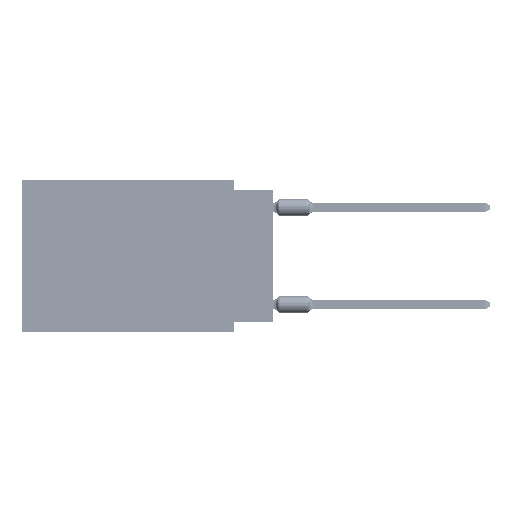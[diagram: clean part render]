
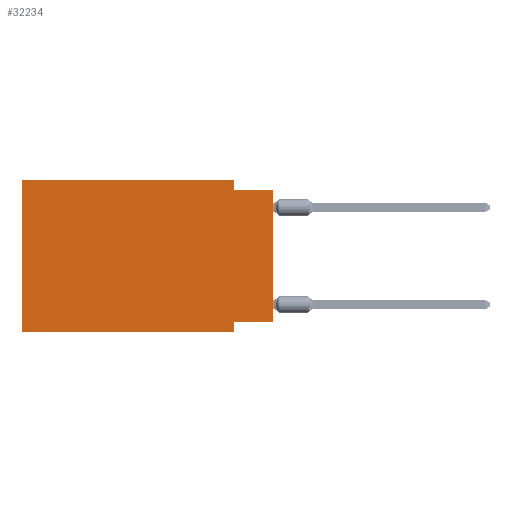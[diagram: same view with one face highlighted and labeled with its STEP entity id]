
A CAD part, left-side view. The second image highlights one B-rep face of the part: STEP entity #32234.
In plain terms, the highlighted planar face has unit normal (-1, 0, 0).
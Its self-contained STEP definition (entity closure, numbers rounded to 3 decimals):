
#1309 = CARTESIAN_POINT ( 'NONE',  ( 0., 2.54, -9.906 ) ) ;
#2368 = ORIENTED_EDGE ( 'NONE', *, *, #72979, .F. ) ;
#2607 = DIRECTION ( 'NONE',  ( 0., 0., -1. ) ) ;
#2869 = VERTEX_POINT ( 'NONE', #23513 ) ;
#4216 = EDGE_CURVE ( 'NONE', #22415, #53746, #67409, .T. ) ;
#5171 = DIRECTION ( 'NONE',  ( 0., 0., -1. ) ) ;
#5966 = CARTESIAN_POINT ( 'NONE',  ( 0., 16.383, -9.906 ) ) ;
#9535 = ORIENTED_EDGE ( 'NONE', *, *, #80196, .F. ) ;
#10734 = VERTEX_POINT ( 'NONE', #16359 ) ;
#12875 = EDGE_CURVE ( 'NONE', #22415, #37363, #29248, .T. ) ;
#15638 = CARTESIAN_POINT ( 'NONE',  ( 0., 2.54, 0. ) ) ;
#16359 = CARTESIAN_POINT ( 'NONE',  ( 0., 0., -0.635 ) ) ;
#18147 = EDGE_CURVE ( 'NONE', #49187, #87806, #49714, .T. ) ;
#18782 = VECTOR ( 'NONE', #42097, 1000. ) ;
#20379 = PLANE ( 'NONE',  #30728 ) ;
#22060 = VECTOR ( 'NONE', #2607, 1000. ) ;
#22415 = VERTEX_POINT ( 'NONE', #23471 ) ;
#23441 = CARTESIAN_POINT ( 'NONE',  ( 0., 2.54, -9.906 ) ) ;
#23471 = CARTESIAN_POINT ( 'NONE',  ( 0., 16.383, -9.906 ) ) ;
#23513 = CARTESIAN_POINT ( 'NONE',  ( 0., 0., -9.271 ) ) ;
#24281 = CARTESIAN_POINT ( 'NONE',  ( 0., 2.54, 0. ) ) ;
#25303 = DIRECTION ( 'NONE',  ( 0., -1., 0. ) ) ;
#26693 = FACE_OUTER_BOUND ( 'NONE', #75995, .T. ) ;
#29152 = ORIENTED_EDGE ( 'NONE', *, *, #18147, .F. ) ;
#29248 = LINE ( 'NONE', #64616, #82178 ) ;
#30728 = AXIS2_PLACEMENT_3D ( 'NONE', #54037, #39248, #5171 ) ;
#30742 = LINE ( 'NONE', #65251, #62306 ) ;
#32234 = ADVANCED_FACE ( 'NONE', ( #26693 ), #20379, .F. ) ;
#34248 = VECTOR ( 'NONE', #83323, 1000. ) ;
#35223 = ORIENTED_EDGE ( 'NONE', *, *, #56813, .T. ) ;
#35950 = DIRECTION ( 'NONE',  ( 0., 0., 1. ) ) ;
#37011 = DIRECTION ( 'NONE',  ( 0., -1., 0. ) ) ;
#37363 = VERTEX_POINT ( 'NONE', #61233 ) ;
#37779 = LINE ( 'NONE', #39539, #55965 ) ;
#39248 = DIRECTION ( 'NONE',  ( 1., 0., 0. ) ) ;
#39539 = CARTESIAN_POINT ( 'NONE',  ( 0., 0., 0. ) ) ;
#42097 = DIRECTION ( 'NONE',  ( 0., -1., 0. ) ) ;
#43469 = LINE ( 'NONE', #1309, #77709 ) ;
#45109 = CARTESIAN_POINT ( 'NONE',  ( 0., 2.54, -0.635 ) ) ;
#45384 = ORIENTED_EDGE ( 'NONE', *, *, #4216, .T. ) ;
#49187 = VERTEX_POINT ( 'NONE', #24281 ) ;
#49706 = CARTESIAN_POINT ( 'NONE',  ( 0., 0., -0.635 ) ) ;
#49714 = LINE ( 'NONE', #15638, #22060 ) ;
#52998 = DIRECTION ( 'NONE',  ( 0., 0., 1. ) ) ;
#53746 = VERTEX_POINT ( 'NONE', #23441 ) ;
#54037 = CARTESIAN_POINT ( 'NONE',  ( 0., 16.383, 0. ) ) ;
#55712 = EDGE_CURVE ( 'NONE', #87806, #10734, #77068, .T. ) ;
#55965 = VECTOR ( 'NONE', #52998, 1000. ) ;
#56813 = EDGE_CURVE ( 'NONE', #2869, #10734, #37779, .T. ) ;
#59453 = VECTOR ( 'NONE', #25303, 1000. ) ;
#61233 = CARTESIAN_POINT ( 'NONE',  ( 0., 16.383, 0. ) ) ;
#62306 = VECTOR ( 'NONE', #37011, 1000. ) ;
#62713 = LINE ( 'NONE', #84209, #34248 ) ;
#64616 = CARTESIAN_POINT ( 'NONE',  ( 0., 16.383, 0. ) ) ;
#65251 = CARTESIAN_POINT ( 'NONE',  ( 0., 16.383, 0. ) ) ;
#67409 = LINE ( 'NONE', #5966, #59453 ) ;
#67891 = ORIENTED_EDGE ( 'NONE', *, *, #12875, .F. ) ;
#72979 = EDGE_CURVE ( 'NONE', #2869, #83261, #62713, .T. ) ;
#74254 = ORIENTED_EDGE ( 'NONE', *, *, #76981, .F. ) ;
#74297 = ORIENTED_EDGE ( 'NONE', *, *, #55712, .F. ) ;
#75995 = EDGE_LOOP ( 'NONE', ( #35223, #74297, #29152, #9535, #67891, #45384, #74254, #2368 ) ) ;
#76754 = CARTESIAN_POINT ( 'NONE',  ( 0., 2.54, -9.271 ) ) ;
#76981 = EDGE_CURVE ( 'NONE', #83261, #53746, #43469, .T. ) ;
#77068 = LINE ( 'NONE', #49706, #18782 ) ;
#77709 = VECTOR ( 'NONE', #83816, 1000. ) ;
#80196 = EDGE_CURVE ( 'NONE', #37363, #49187, #30742, .T. ) ;
#82178 = VECTOR ( 'NONE', #35950, 1000. ) ;
#83261 = VERTEX_POINT ( 'NONE', #76754 ) ;
#83323 = DIRECTION ( 'NONE',  ( 0., 1., 0. ) ) ;
#83816 = DIRECTION ( 'NONE',  ( 0., 0., -1. ) ) ;
#84209 = CARTESIAN_POINT ( 'NONE',  ( 0., 0., -9.271 ) ) ;
#87806 = VERTEX_POINT ( 'NONE', #45109 ) ;
